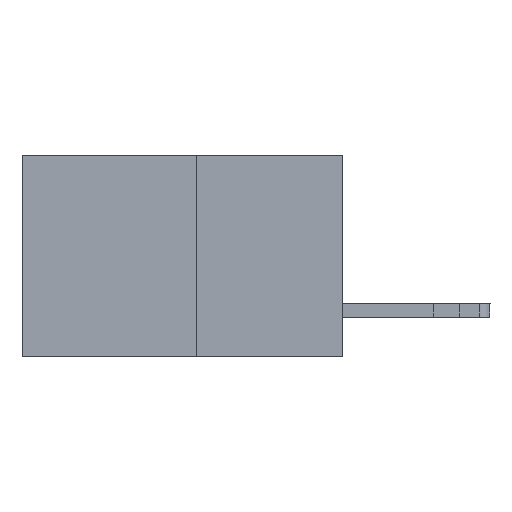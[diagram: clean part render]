
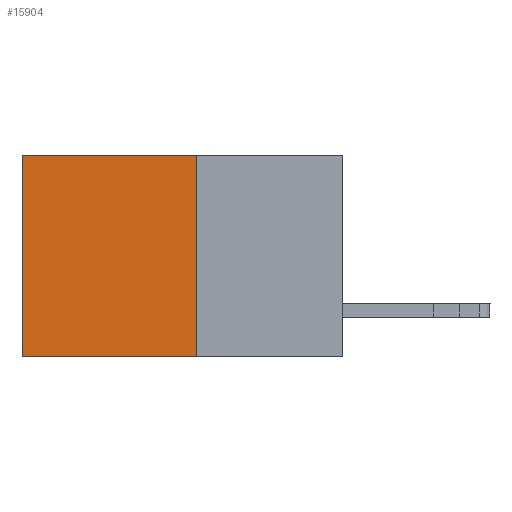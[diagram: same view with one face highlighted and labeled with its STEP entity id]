
A CAD part, left-side view. The second image highlights one B-rep face of the part: STEP entity #15904.
In plain terms, the highlighted planar face has unit normal (-1, 0, 0).
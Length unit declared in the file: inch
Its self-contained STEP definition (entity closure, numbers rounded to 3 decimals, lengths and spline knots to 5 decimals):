
#368 = LINE ( 'NONE', #8966, #5362 ) ;
#418 = CARTESIAN_POINT ( 'NONE',  ( 0.277, 0.27, 0. ) ) ;
#493 = VECTOR ( 'NONE', #12361, 39.37008 ) ;
#1788 = VECTOR ( 'NONE', #2069, 39.37008 ) ;
#2069 = DIRECTION ( 'NONE',  ( 0., 1., 0. ) ) ;
#2862 = EDGE_CURVE ( 'NONE', #9609, #26239, #368, .T. ) ;
#3200 = CARTESIAN_POINT ( 'NONE',  ( 0.277, 0.59, -0.37 ) ) ;
#3960 = LINE ( 'NONE', #3200, #14763 ) ;
#4152 = VERTEX_POINT ( 'NONE', #418 ) ;
#5362 = VECTOR ( 'NONE', #20385, 39.37008 ) ;
#5807 = CARTESIAN_POINT ( 'NONE',  ( 0.277, 0.27, -0.37 ) ) ;
#7495 = DIRECTION ( 'NONE',  ( 0., 0., -1. ) ) ;
#7894 = ORIENTED_EDGE ( 'NONE', *, *, #23372, .T. ) ;
#8129 = LINE ( 'NONE', #27852, #1788 ) ;
#8267 = CARTESIAN_POINT ( 'NONE',  ( 0.277, 0.27, -0.37 ) ) ;
#8966 = CARTESIAN_POINT ( 'NONE',  ( 0.277, 0.27, -0.37 ) ) ;
#9609 = VERTEX_POINT ( 'NONE', #5807 ) ;
#10210 = AXIS2_PLACEMENT_3D ( 'NONE', #8267, #23478, #10508 ) ;
#10508 = DIRECTION ( 'NONE',  ( 0., 0., -1. ) ) ;
#12361 = DIRECTION ( 'NONE',  ( 0., 0., -1. ) ) ;
#12477 = VERTEX_POINT ( 'NONE', #13144 ) ;
#13144 = CARTESIAN_POINT ( 'NONE',  ( 0.277, 0.59, 0. ) ) ;
#14763 = VECTOR ( 'NONE', #7495, 39.37008 ) ;
#15904 = ADVANCED_FACE ( 'NONE', ( #27525 ), #27644, .F. ) ;
#16069 = EDGE_LOOP ( 'NONE', ( #16450, #27437, #25216, #7894 ) ) ;
#16450 = ORIENTED_EDGE ( 'NONE', *, *, #26054, .T. ) ;
#17020 = LINE ( 'NONE', #25318, #493 ) ;
#20385 = DIRECTION ( 'NONE',  ( 0., 1., 0. ) ) ;
#21169 = CARTESIAN_POINT ( 'NONE',  ( 0.277, 0.59, -0.37 ) ) ;
#22556 = EDGE_CURVE ( 'NONE', #4152, #9609, #17020, .T. ) ;
#23372 = EDGE_CURVE ( 'NONE', #4152, #12477, #8129, .T. ) ;
#23478 = DIRECTION ( 'NONE',  ( 1., 0., 0. ) ) ;
#25216 = ORIENTED_EDGE ( 'NONE', *, *, #22556, .F. ) ;
#25318 = CARTESIAN_POINT ( 'NONE',  ( 0.277, 0.27, -0.37 ) ) ;
#26054 = EDGE_CURVE ( 'NONE', #12477, #26239, #3960, .T. ) ;
#26239 = VERTEX_POINT ( 'NONE', #21169 ) ;
#27437 = ORIENTED_EDGE ( 'NONE', *, *, #2862, .F. ) ;
#27525 = FACE_OUTER_BOUND ( 'NONE', #16069, .T. ) ;
#27644 = PLANE ( 'NONE',  #10210 ) ;
#27852 = CARTESIAN_POINT ( 'NONE',  ( 0.277, 0.27, 0. ) ) ;
